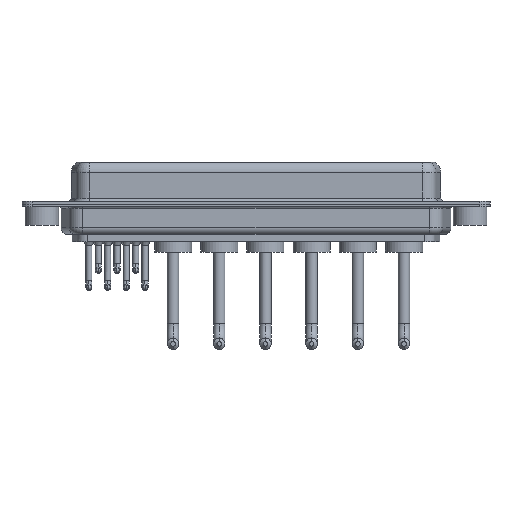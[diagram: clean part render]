
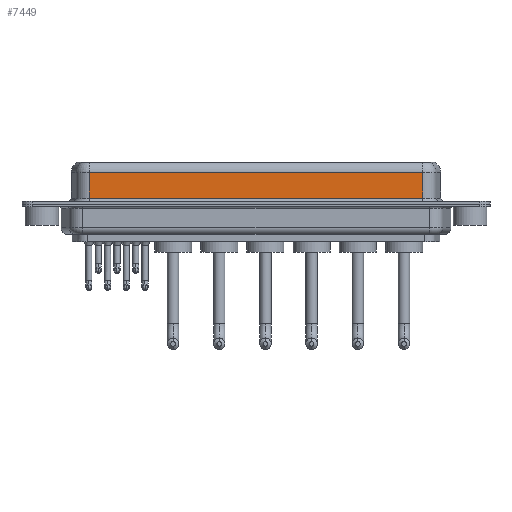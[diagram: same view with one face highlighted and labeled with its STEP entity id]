
A CAD part, front view. The second image highlights one B-rep face of the part: STEP entity #7449.
In plain terms, the highlighted planar face has unit normal (0, -1, 0).
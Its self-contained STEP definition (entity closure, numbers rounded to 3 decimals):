
#572 = EDGE_CURVE ( 'NONE', #3944, #2960, #11254, .T. ) ;
#1171 = VECTOR ( 'NONE', #15515, 1000. ) ;
#1561 = VECTOR ( 'NONE', #6868, 1000. ) ;
#2669 = EDGE_LOOP ( 'NONE', ( #13170, #12510, #15076, #9815 ) ) ;
#2960 = VERTEX_POINT ( 'NONE', #3924 ) ;
#3363 = VECTOR ( 'NONE', #15387, 1000. ) ;
#3924 = CARTESIAN_POINT ( 'NONE',  ( 56.462, -3.95, 0.9 ) ) ;
#3944 = VERTEX_POINT ( 'NONE', #7759 ) ;
#3973 = DIRECTION ( 'NONE',  ( 0., 0., 1. ) ) ;
#4725 = CARTESIAN_POINT ( 'NONE',  ( 7.038, -3.95, 4.65 ) ) ;
#5913 = LINE ( 'NONE', #12632, #12501 ) ;
#6016 = AXIS2_PLACEMENT_3D ( 'NONE', #10784, #15358, #3973 ) ;
#6868 = DIRECTION ( 'NONE',  ( 1., 0., 0. ) ) ;
#7449 = ADVANCED_FACE ( 'NONE', ( #18387 ), #18296, .F. ) ;
#7759 = CARTESIAN_POINT ( 'NONE',  ( 7.038, -3.95, 0.9 ) ) ;
#8389 = VERTEX_POINT ( 'NONE', #4725 ) ;
#8543 = CARTESIAN_POINT ( 'NONE',  ( 56.462, -3.95, 6.4 ) ) ;
#9746 = LINE ( 'NONE', #8543, #1171 ) ;
#9815 = ORIENTED_EDGE ( 'NONE', *, *, #572, .T. ) ;
#10754 = VERTEX_POINT ( 'NONE', #12895 ) ;
#10784 = CARTESIAN_POINT ( 'NONE',  ( 56.462, -3.95, 6.4 ) ) ;
#11254 = LINE ( 'NONE', #16967, #1561 ) ;
#11913 = EDGE_CURVE ( 'NONE', #10754, #2960, #9746, .T. ) ;
#12501 = VECTOR ( 'NONE', #15432, 1000. ) ;
#12510 = ORIENTED_EDGE ( 'NONE', *, *, #17029, .T. ) ;
#12554 = EDGE_CURVE ( 'NONE', #8389, #3944, #5913, .T. ) ;
#12632 = CARTESIAN_POINT ( 'NONE',  ( 7.038, -3.95, 6.4 ) ) ;
#12895 = CARTESIAN_POINT ( 'NONE',  ( 56.462, -3.95, 4.65 ) ) ;
#13170 = ORIENTED_EDGE ( 'NONE', *, *, #11913, .F. ) ;
#15076 = ORIENTED_EDGE ( 'NONE', *, *, #12554, .T. ) ;
#15298 = LINE ( 'NONE', #15477, #3363 ) ;
#15358 = DIRECTION ( 'NONE',  ( 0., 1., 0. ) ) ;
#15387 = DIRECTION ( 'NONE',  ( -1., 0., 0. ) ) ;
#15432 = DIRECTION ( 'NONE',  ( 0., 0., -1. ) ) ;
#15477 = CARTESIAN_POINT ( 'NONE',  ( 56.462, -3.95, 4.65 ) ) ;
#15515 = DIRECTION ( 'NONE',  ( 0., 0., -1. ) ) ;
#16967 = CARTESIAN_POINT ( 'NONE',  ( 56.462, -3.95, 0.9 ) ) ;
#17029 = EDGE_CURVE ( 'NONE', #10754, #8389, #15298, .T. ) ;
#18296 = PLANE ( 'NONE',  #6016 ) ;
#18387 = FACE_OUTER_BOUND ( 'NONE', #2669, .T. ) ;
